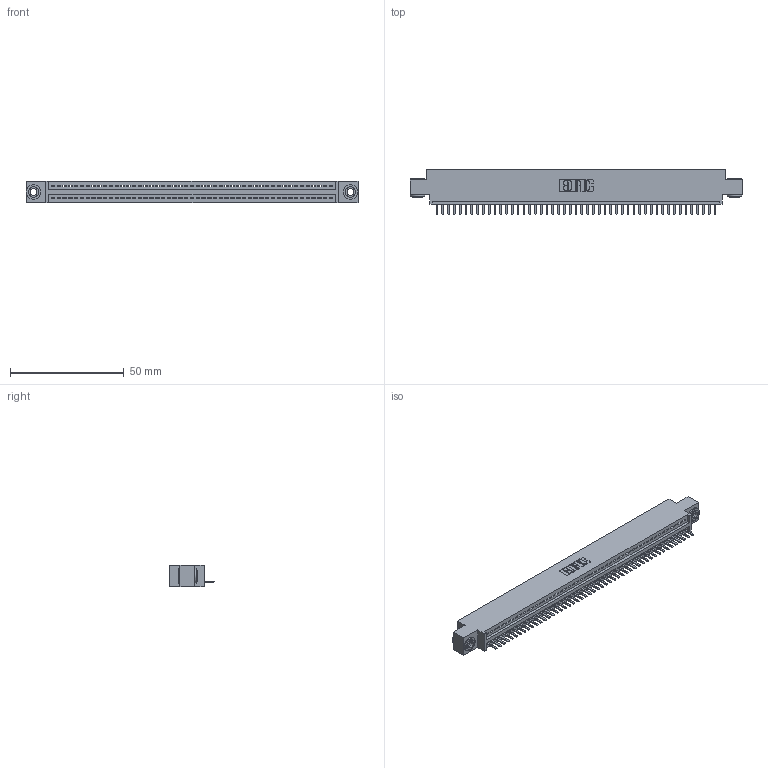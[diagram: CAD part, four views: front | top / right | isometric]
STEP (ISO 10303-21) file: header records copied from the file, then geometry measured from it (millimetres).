
FILE_DESCRIPTION (( 'STEP AP203' ), '1' );
FILE_NAME ('395-049-520-603.STEP', '2018-11-20T01:07:41', ( '' ), ( '' ), 'SwSTEP 2.0', 'SolidWorks 2016', '' );
FILE_SCHEMA (( 'CONFIG_CONTROL_DESIGN' ));
Length unit declared in the file: inch
Products named in the file (4): 345-250-002_345-250-002-102; 345 Part_0.170 Offset - 0.156 Dia-TH; 395-049-520-603; 345-292-001_345-293-120
Assembly tree (52 placements, depth 2):
  395-049-520-603
    345 Part_0.170 Offset - 0.156 Dia-TH
    345-292-001_345-293-120  x49
    345-250-002_345-250-002-102  x2
Bounding box: 145.67 x 19.68 x 9.4 mm (x, y, z)
Volume: 13658.2 mm3; surface area: 18125.6 mm2
Topology: 52 solids, 52 shells, 3206 faces, 9445 edges, 6162 vertices
Faces by surface type: plane 2152, cylinder 1046, cone 8
Entity records: 36832 total; most frequent: CARTESIAN_POINT 6370, ORIENTED_EDGE 6334, DIRECTION 5571, EDGE_CURVE 3167, LINE 2811, VECTOR 2811, VERTEX_POINT 2106, AXIS2_PLACEMENT_3D 1380
